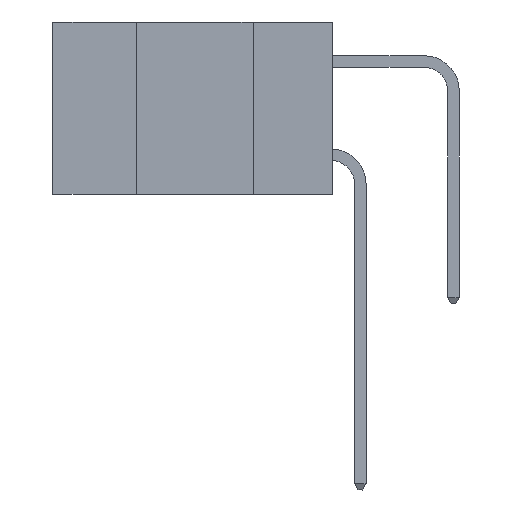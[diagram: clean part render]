
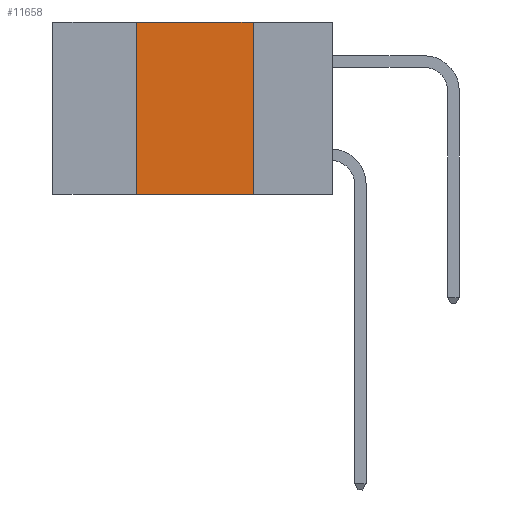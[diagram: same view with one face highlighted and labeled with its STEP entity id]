
A CAD part, left-side view. The second image highlights one B-rep face of the part: STEP entity #11658.
In plain terms, the highlighted planar face has unit normal (-1, 0, 0).
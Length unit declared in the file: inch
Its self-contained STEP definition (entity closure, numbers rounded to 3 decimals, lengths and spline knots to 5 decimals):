
#13 = ORIENTED_EDGE ( 'NONE', *, *, #2736, .F. ) ;
#415 = DIRECTION ( 'NONE',  ( 0., 0., -1. ) ) ;
#617 = EDGE_CURVE ( 'NONE', #9574, #9897, #10192, .T. ) ;
#781 = VECTOR ( 'NONE', #7411, 39.37008 ) ;
#1554 = EDGE_LOOP ( 'NONE', ( #4517, #13, #5141, #8199 ) ) ;
#1612 = CARTESIAN_POINT ( 'NONE',  ( 0., 0.42, 0. ) ) ;
#2535 = EDGE_CURVE ( 'NONE', #9574, #3832, #5679, .T. ) ;
#2736 = EDGE_CURVE ( 'NONE', #3832, #9326, #6077, .T. ) ;
#2966 = VECTOR ( 'NONE', #3896, 39.37008 ) ;
#3143 = LINE ( 'NONE', #7618, #781 ) ;
#3375 = VECTOR ( 'NONE', #5219, 39.37008 ) ;
#3832 = VERTEX_POINT ( 'NONE', #11562 ) ;
#3896 = DIRECTION ( 'NONE',  ( 0., -1., 0. ) ) ;
#4330 = PLANE ( 'NONE',  #5390 ) ;
#4517 = ORIENTED_EDGE ( 'NONE', *, *, #6677, .F. ) ;
#4733 = CARTESIAN_POINT ( 'NONE',  ( 0., 0.6, 0. ) ) ;
#5141 = ORIENTED_EDGE ( 'NONE', *, *, #2535, .F. ) ;
#5219 = DIRECTION ( 'NONE',  ( 0., -1., 0. ) ) ;
#5390 = AXIS2_PLACEMENT_3D ( 'NONE', #6976, #6135, #415 ) ;
#5679 = LINE ( 'NONE', #1612, #8336 ) ;
#5975 = CARTESIAN_POINT ( 'NONE',  ( 0., 0.6, -0.37 ) ) ;
#6077 = LINE ( 'NONE', #4733, #3375 ) ;
#6135 = DIRECTION ( 'NONE',  ( 1., 0., 0. ) ) ;
#6385 = CARTESIAN_POINT ( 'NONE',  ( 0., 0.42, -0.37 ) ) ;
#6677 = EDGE_CURVE ( 'NONE', #9326, #9897, #3143, .T. ) ;
#6976 = CARTESIAN_POINT ( 'NONE',  ( 0., 0.6, 0. ) ) ;
#7411 = DIRECTION ( 'NONE',  ( 0., 0., -1. ) ) ;
#7618 = CARTESIAN_POINT ( 'NONE',  ( 0., 0.17, 0. ) ) ;
#7621 = DIRECTION ( 'NONE',  ( 0., 0., 1. ) ) ;
#8199 = ORIENTED_EDGE ( 'NONE', *, *, #617, .T. ) ;
#8336 = VECTOR ( 'NONE', #7621, 39.37008 ) ;
#8697 = FACE_OUTER_BOUND ( 'NONE', #1554, .T. ) ;
#9326 = VERTEX_POINT ( 'NONE', #11334 ) ;
#9574 = VERTEX_POINT ( 'NONE', #6385 ) ;
#9897 = VERTEX_POINT ( 'NONE', #10377 ) ;
#10192 = LINE ( 'NONE', #5975, #2966 ) ;
#10377 = CARTESIAN_POINT ( 'NONE',  ( 0., 0.17, -0.37 ) ) ;
#11334 = CARTESIAN_POINT ( 'NONE',  ( 0., 0.17, 0. ) ) ;
#11562 = CARTESIAN_POINT ( 'NONE',  ( 0., 0.42, 0. ) ) ;
#11658 = ADVANCED_FACE ( 'NONE', ( #8697 ), #4330, .F. ) ;
